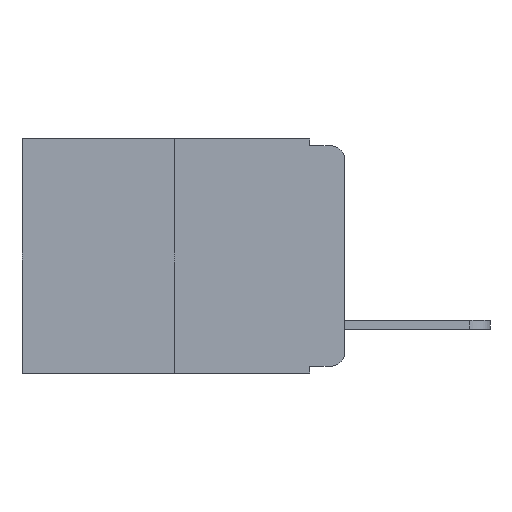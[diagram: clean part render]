
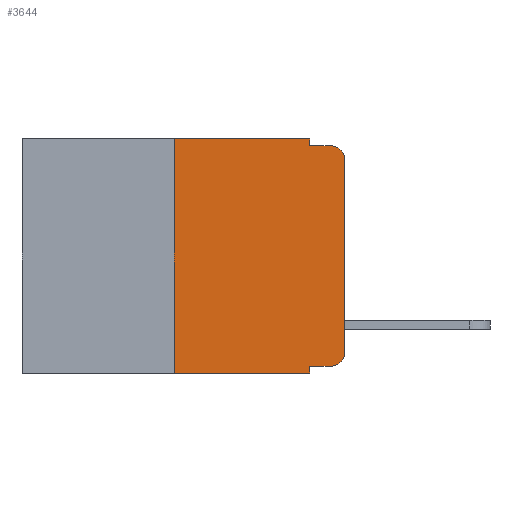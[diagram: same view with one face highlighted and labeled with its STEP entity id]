
A CAD part, left-side view. The second image highlights one B-rep face of the part: STEP entity #3644.
In plain terms, the highlighted planar face has unit normal (-1, 0, 0).
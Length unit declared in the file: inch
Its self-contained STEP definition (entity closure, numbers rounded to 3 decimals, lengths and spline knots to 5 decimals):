
#48 = CARTESIAN_POINT ( 'NONE',  ( 0., 0.02, -0.01 ) ) ;
#119 = VERTEX_POINT ( 'NONE', #48 ) ;
#219 = AXIS2_PLACEMENT_3D ( 'NONE', #4781, #7799, #672 ) ;
#672 = DIRECTION ( 'NONE',  ( 0., 0., -1. ) ) ;
#971 = DIRECTION ( 'NONE',  ( 0., -1., 0. ) ) ;
#1207 = CARTESIAN_POINT ( 'NONE',  ( 0., 0.051, -0.343 ) ) ;
#1291 = VECTOR ( 'NONE', #8735, 39.37008 ) ;
#1366 = DIRECTION ( 'NONE',  ( 0., 0., -1. ) ) ;
#1470 = FACE_OUTER_BOUND ( 'NONE', #5003, .T. ) ;
#1796 = VERTEX_POINT ( 'NONE', #6253 ) ;
#1847 = CARTESIAN_POINT ( 'NONE',  ( 0., 0.473, 0. ) ) ;
#1929 = ORIENTED_EDGE ( 'NONE', *, *, #5939, .F. ) ;
#1964 = VECTOR ( 'NONE', #971, 39.37008 ) ;
#1984 = VECTOR ( 'NONE', #1366, 39.37008 ) ;
#2086 = VECTOR ( 'NONE', #6150, 39.37008 ) ;
#2104 = ORIENTED_EDGE ( 'NONE', *, *, #8303, .T. ) ;
#2417 = CARTESIAN_POINT ( 'NONE',  ( 0., 0.051, 0. ) ) ;
#2492 = DIRECTION ( 'NONE',  ( 0., 0., 1. ) ) ;
#2583 = LINE ( 'NONE', #13622, #13674 ) ;
#2759 = ORIENTED_EDGE ( 'NONE', *, *, #4392, .T. ) ;
#2888 = DIRECTION ( 'NONE',  ( 1., 0., 0. ) ) ;
#2983 = EDGE_CURVE ( 'NONE', #12380, #119, #8479, .T. ) ;
#3221 = CARTESIAN_POINT ( 'NONE',  ( 0., 0.051, 0. ) ) ;
#3644 = ADVANCED_FACE ( 'NONE', ( #1470 ), #10397, .F. ) ;
#3685 = AXIS2_PLACEMENT_3D ( 'NONE', #13349, #10231, #10327 ) ;
#3730 = EDGE_CURVE ( 'NONE', #4360, #7545, #12425, .T. ) ;
#3945 = DIRECTION ( 'NONE',  ( 0., -1., 0. ) ) ;
#4151 = LINE ( 'NONE', #8874, #1291 ) ;
#4306 = VERTEX_POINT ( 'NONE', #10597 ) ;
#4360 = VERTEX_POINT ( 'NONE', #5383 ) ;
#4392 = EDGE_CURVE ( 'NONE', #4306, #13348, #4151, .T. ) ;
#4566 = CARTESIAN_POINT ( 'NONE',  ( 0., 0., -0.313 ) ) ;
#4781 = CARTESIAN_POINT ( 'NONE',  ( 0., 0.02, -0.313 ) ) ;
#5003 = EDGE_LOOP ( 'NONE', ( #10391, #10483, #1929, #10465, #13127, #12985, #2759, #13430, #10693, #2104 ) ) ;
#5123 = CARTESIAN_POINT ( 'NONE',  ( 0., 0.25, 0. ) ) ;
#5307 = LINE ( 'NONE', #11360, #2086 ) ;
#5383 = CARTESIAN_POINT ( 'NONE',  ( 0., 0.051, -0.333 ) ) ;
#5939 = EDGE_CURVE ( 'NONE', #1796, #119, #2583, .T. ) ;
#6150 = DIRECTION ( 'NONE',  ( 0., 0., 1. ) ) ;
#6163 = DIRECTION ( 'NONE',  ( 0., 0., -1. ) ) ;
#6253 = CARTESIAN_POINT ( 'NONE',  ( 0., 0.051, -0.01 ) ) ;
#6304 = CARTESIAN_POINT ( 'NONE',  ( 0., 0., -0.03 ) ) ;
#6392 = CARTESIAN_POINT ( 'NONE',  ( 0., 0.051, -0.333 ) ) ;
#6423 = EDGE_CURVE ( 'NONE', #12888, #10341, #11201, .T. ) ;
#6674 = EDGE_CURVE ( 'NONE', #10341, #1796, #9373, .T. ) ;
#6843 = EDGE_CURVE ( 'NONE', #10024, #12380, #11431, .T. ) ;
#7219 = VECTOR ( 'NONE', #7491, 39.37008 ) ;
#7491 = DIRECTION ( 'NONE',  ( 0., 0., -1. ) ) ;
#7545 = VERTEX_POINT ( 'NONE', #12955 ) ;
#7751 = CARTESIAN_POINT ( 'NONE',  ( 0., 0.051, 0. ) ) ;
#7799 = DIRECTION ( 'NONE',  ( -1., 0., 0. ) ) ;
#8123 = EDGE_CURVE ( 'NONE', #4360, #13348, #11129, .T. ) ;
#8294 = AXIS2_PLACEMENT_3D ( 'NONE', #1847, #2888, #6163 ) ;
#8303 = EDGE_CURVE ( 'NONE', #7545, #10024, #13572, .T. ) ;
#8479 = CIRCLE ( 'NONE', #3685, 0.02 ) ;
#8735 = DIRECTION ( 'NONE',  ( 0., -1., 0. ) ) ;
#8874 = CARTESIAN_POINT ( 'NONE',  ( 0., 0.473, -0.343 ) ) ;
#9373 = LINE ( 'NONE', #3221, #7219 ) ;
#10024 = VERTEX_POINT ( 'NONE', #4566 ) ;
#10175 = DIRECTION ( 'NONE',  ( 0., -1., 0. ) ) ;
#10231 = DIRECTION ( 'NONE',  ( -1., 0., 0. ) ) ;
#10327 = DIRECTION ( 'NONE',  ( 0., 0., -1. ) ) ;
#10341 = VERTEX_POINT ( 'NONE', #2417 ) ;
#10391 = ORIENTED_EDGE ( 'NONE', *, *, #6843, .T. ) ;
#10397 = PLANE ( 'NONE',  #8294 ) ;
#10465 = ORIENTED_EDGE ( 'NONE', *, *, #6674, .F. ) ;
#10483 = ORIENTED_EDGE ( 'NONE', *, *, #2983, .T. ) ;
#10597 = CARTESIAN_POINT ( 'NONE',  ( 0., 0.25, -0.343 ) ) ;
#10693 = ORIENTED_EDGE ( 'NONE', *, *, #3730, .T. ) ;
#11089 = VECTOR ( 'NONE', #2492, 39.37008 ) ;
#11129 = LINE ( 'NONE', #7751, #1984 ) ;
#11201 = LINE ( 'NONE', #13432, #12660 ) ;
#11360 = CARTESIAN_POINT ( 'NONE',  ( 0., 0.25, 0. ) ) ;
#11431 = LINE ( 'NONE', #12005, #11089 ) ;
#12005 = CARTESIAN_POINT ( 'NONE',  ( 0., 0., 0. ) ) ;
#12380 = VERTEX_POINT ( 'NONE', #6304 ) ;
#12425 = LINE ( 'NONE', #6392, #1964 ) ;
#12660 = VECTOR ( 'NONE', #10175, 39.37008 ) ;
#12888 = VERTEX_POINT ( 'NONE', #5123 ) ;
#12955 = CARTESIAN_POINT ( 'NONE',  ( 0., 0.02, -0.333 ) ) ;
#12985 = ORIENTED_EDGE ( 'NONE', *, *, #12992, .F. ) ;
#12992 = EDGE_CURVE ( 'NONE', #4306, #12888, #5307, .T. ) ;
#13127 = ORIENTED_EDGE ( 'NONE', *, *, #6423, .F. ) ;
#13348 = VERTEX_POINT ( 'NONE', #1207 ) ;
#13349 = CARTESIAN_POINT ( 'NONE',  ( 0., 0.02, -0.03 ) ) ;
#13430 = ORIENTED_EDGE ( 'NONE', *, *, #8123, .F. ) ;
#13432 = CARTESIAN_POINT ( 'NONE',  ( 0., 0.473, 0. ) ) ;
#13572 = CIRCLE ( 'NONE', #219, 0.02 ) ;
#13622 = CARTESIAN_POINT ( 'NONE',  ( 0., 0.051, -0.01 ) ) ;
#13674 = VECTOR ( 'NONE', #3945, 39.37008 ) ;
